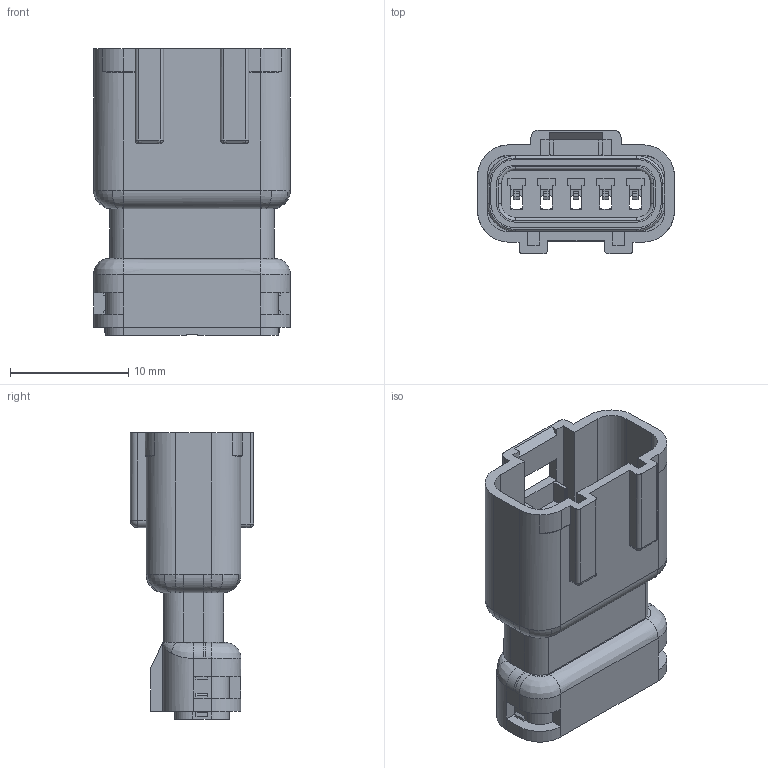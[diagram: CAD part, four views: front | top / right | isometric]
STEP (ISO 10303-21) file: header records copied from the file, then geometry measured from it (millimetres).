
FILE_DESCRIPTION (( 'STEP AP214' ), '1' );
FILE_NAME ('565-005-000-311.STEP', '2020-07-27T15:54:41', ( '' ), ( '' ), 'SwSTEP 2.0', 'SolidWorks 2020', '' );
FILE_SCHEMA (( 'AUTOMOTIVE_DESIGN' ));
Length unit declared in the file: millimetre
Products named in the file (5): 565-005-000-311; 565-005-000-311_Housing; 565-005-000-311_Rear Gasket; 565-005-000-311_Front Gasket; 565-005-000-311_Rear Insulator
Assembly tree (4 placements, depth 2):
  565-005-000-311
    565-005-000-311_Housing
    565-005-000-311_Rear Insulator
    565-005-000-311_Rear Gasket
    565-005-000-311_Front Gasket
Bounding box: 16.6 x 10.4 x 24.18 mm (x, y, z)
Volume: 1481.8 mm3; surface area: 3614.5 mm2
Topology: 4 solids, 4 shells, 653 faces, 1764 edges, 1140 vertices
Faces by surface type: plane 376, cylinder 171, bspline 58, torus 42, sphere 6
Entity records: 22190 total; most frequent: CARTESIAN_POINT 5761, ORIENTED_EDGE 3516, DIRECTION 3242, EDGE_CURVE 1758, VECTOR 1144, LINE 1144, VERTEX_POINT 1140, AXIS2_PLACEMENT_3D 1049
